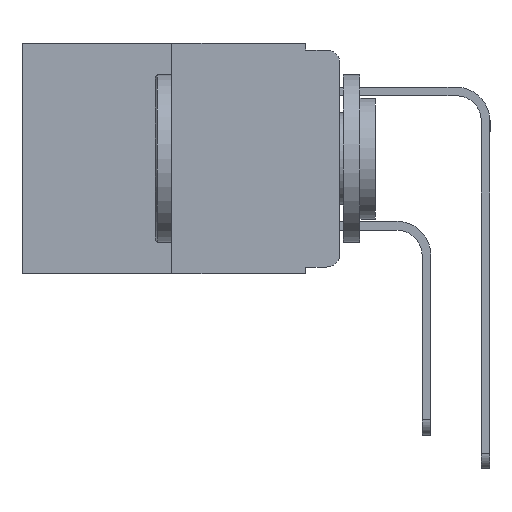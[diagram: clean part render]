
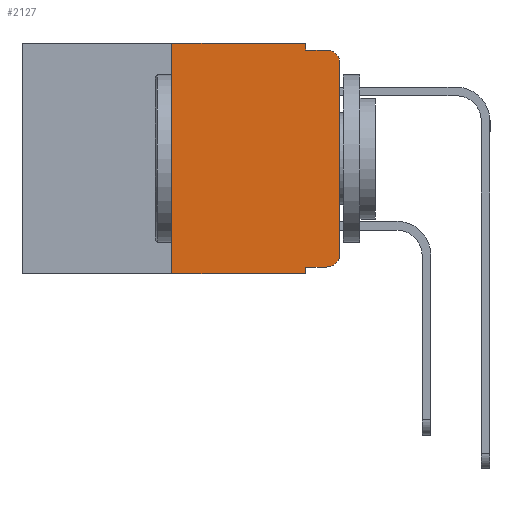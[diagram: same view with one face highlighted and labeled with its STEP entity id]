
A CAD part, left-side view. The second image highlights one B-rep face of the part: STEP entity #2127.
In plain terms, the highlighted planar face has unit normal (-1, 0, 0).
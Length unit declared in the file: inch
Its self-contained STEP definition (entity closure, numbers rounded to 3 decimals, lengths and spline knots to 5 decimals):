
#459 = VECTOR ( 'NONE', #6215, 39.37008 ) ;
#470 = VECTOR ( 'NONE', #4532, 39.37008 ) ;
#555 = EDGE_CURVE ( 'NONE', #13656, #2213, #9569, .T. ) ;
#850 = VECTOR ( 'NONE', #9833, 39.37008 ) ;
#875 = DIRECTION ( 'NONE',  ( 0., 0., -1. ) ) ;
#963 = DIRECTION ( 'NONE',  ( 0., 0., -1. ) ) ;
#992 = CARTESIAN_POINT ( 'NONE',  ( 0., 0.051, -0.01 ) ) ;
#1230 = ORIENTED_EDGE ( 'NONE', *, *, #10964, .F. ) ;
#1319 = ORIENTED_EDGE ( 'NONE', *, *, #9535, .T. ) ;
#1348 = ORIENTED_EDGE ( 'NONE', *, *, #10260, .F. ) ;
#1674 = LINE ( 'NONE', #11668, #7772 ) ;
#1982 = AXIS2_PLACEMENT_3D ( 'NONE', #13988, #7801, #875 ) ;
#2127 = ADVANCED_FACE ( 'NONE', ( #6171 ), #11903, .F. ) ;
#2213 = VERTEX_POINT ( 'NONE', #8237 ) ;
#2452 = LINE ( 'NONE', #5250, #13628 ) ;
#2521 = CARTESIAN_POINT ( 'NONE',  ( 0., 0.051, -0.333 ) ) ;
#2648 = ORIENTED_EDGE ( 'NONE', *, *, #555, .T. ) ;
#2690 = ORIENTED_EDGE ( 'NONE', *, *, #8818, .T. ) ;
#2891 = VERTEX_POINT ( 'NONE', #10440 ) ;
#2963 = VERTEX_POINT ( 'NONE', #10147 ) ;
#3169 = CARTESIAN_POINT ( 'NONE',  ( 0., 0.473, 0. ) ) ;
#3643 = VERTEX_POINT ( 'NONE', #12414 ) ;
#3748 = AXIS2_PLACEMENT_3D ( 'NONE', #14054, #7883, #963 ) ;
#4174 = CARTESIAN_POINT ( 'NONE',  ( 0., 0., -0.313 ) ) ;
#4399 = LINE ( 'NONE', #3169, #850 ) ;
#4422 = LINE ( 'NONE', #6981, #7045 ) ;
#4532 = DIRECTION ( 'NONE',  ( 0., -1., 0. ) ) ;
#4603 = CARTESIAN_POINT ( 'NONE',  ( 0., 0.25, 0. ) ) ;
#4825 = CARTESIAN_POINT ( 'NONE',  ( 0., 0.02, -0.333 ) ) ;
#4861 = ORIENTED_EDGE ( 'NONE', *, *, #12292, .F. ) ;
#5182 = DIRECTION ( 'NONE',  ( 0., 0., -1. ) ) ;
#5250 = CARTESIAN_POINT ( 'NONE',  ( 0., 0.051, -0.333 ) ) ;
#5542 = ORIENTED_EDGE ( 'NONE', *, *, #12956, .T. ) ;
#5686 = EDGE_LOOP ( 'NONE', ( #6267, #5542, #4861, #9204, #11367, #1230, #2648, #1348, #1319, #2690 ) ) ;
#5704 = CARTESIAN_POINT ( 'NONE',  ( 0., 0.473, -0.343 ) ) ;
#5944 = AXIS2_PLACEMENT_3D ( 'NONE', #9062, #13264, #13259 ) ;
#6120 = DIRECTION ( 'NONE',  ( 0., 0., 1. ) ) ;
#6171 = FACE_OUTER_BOUND ( 'NONE', #5686, .T. ) ;
#6215 = DIRECTION ( 'NONE',  ( 0., -1., 0. ) ) ;
#6267 = ORIENTED_EDGE ( 'NONE', *, *, #13649, .T. ) ;
#6360 = VERTEX_POINT ( 'NONE', #4174 ) ;
#6499 = DIRECTION ( 'NONE',  ( 0., 0., 1. ) ) ;
#6612 = VERTEX_POINT ( 'NONE', #4603 ) ;
#6735 = VERTEX_POINT ( 'NONE', #2521 ) ;
#6981 = CARTESIAN_POINT ( 'NONE',  ( 0., 0.051, 0. ) ) ;
#7045 = VECTOR ( 'NONE', #11262, 39.37008 ) ;
#7772 = VECTOR ( 'NONE', #5182, 39.37008 ) ;
#7801 = DIRECTION ( 'NONE',  ( -1., 0., 0. ) ) ;
#7883 = DIRECTION ( 'NONE',  ( -1., 0., 0. ) ) ;
#8237 = CARTESIAN_POINT ( 'NONE',  ( 0., 0.051, -0.343 ) ) ;
#8638 = CARTESIAN_POINT ( 'NONE',  ( 0., 0., -0.03 ) ) ;
#8808 = CIRCLE ( 'NONE', #3748, 0.02 ) ;
#8818 = EDGE_CURVE ( 'NONE', #10871, #6360, #8808, .T. ) ;
#8891 = CIRCLE ( 'NONE', #1982, 0.02 ) ;
#9062 = CARTESIAN_POINT ( 'NONE',  ( 0., 0.473, 0. ) ) ;
#9204 = ORIENTED_EDGE ( 'NONE', *, *, #11642, .F. ) ;
#9535 = EDGE_CURVE ( 'NONE', #6735, #10871, #2452, .T. ) ;
#9569 = LINE ( 'NONE', #5704, #459 ) ;
#9833 = DIRECTION ( 'NONE',  ( 0., -1., 0. ) ) ;
#10147 = CARTESIAN_POINT ( 'NONE',  ( 0., 0.02, -0.01 ) ) ;
#10260 = EDGE_CURVE ( 'NONE', #6735, #2213, #1674, .T. ) ;
#10440 = CARTESIAN_POINT ( 'NONE',  ( 0., 0.051, -0.01 ) ) ;
#10460 = CARTESIAN_POINT ( 'NONE',  ( 0., 0.25, 0. ) ) ;
#10871 = VERTEX_POINT ( 'NONE', #4825 ) ;
#10964 = EDGE_CURVE ( 'NONE', #13656, #6612, #13276, .T. ) ;
#11193 = VERTEX_POINT ( 'NONE', #8638 ) ;
#11224 = VECTOR ( 'NONE', #6499, 39.37008 ) ;
#11262 = DIRECTION ( 'NONE',  ( 0., 0., -1. ) ) ;
#11367 = ORIENTED_EDGE ( 'NONE', *, *, #12884, .F. ) ;
#11543 = LINE ( 'NONE', #11844, #11224 ) ;
#11642 = EDGE_CURVE ( 'NONE', #3643, #2891, #4422, .T. ) ;
#11668 = CARTESIAN_POINT ( 'NONE',  ( 0., 0.051, 0. ) ) ;
#11723 = DIRECTION ( 'NONE',  ( 0., -1., 0. ) ) ;
#11844 = CARTESIAN_POINT ( 'NONE',  ( 0., 0., 0. ) ) ;
#11903 = PLANE ( 'NONE',  #5944 ) ;
#12292 = EDGE_CURVE ( 'NONE', #2891, #2963, #12310, .T. ) ;
#12310 = LINE ( 'NONE', #992, #470 ) ;
#12414 = CARTESIAN_POINT ( 'NONE',  ( 0., 0.051, 0. ) ) ;
#12836 = CARTESIAN_POINT ( 'NONE',  ( 0., 0.25, -0.343 ) ) ;
#12884 = EDGE_CURVE ( 'NONE', #6612, #3643, #4399, .T. ) ;
#12956 = EDGE_CURVE ( 'NONE', #11193, #2963, #8891, .T. ) ;
#12959 = VECTOR ( 'NONE', #6120, 39.37008 ) ;
#13259 = DIRECTION ( 'NONE',  ( 0., 0., -1. ) ) ;
#13264 = DIRECTION ( 'NONE',  ( 1., 0., 0. ) ) ;
#13276 = LINE ( 'NONE', #10460, #12959 ) ;
#13628 = VECTOR ( 'NONE', #11723, 39.37008 ) ;
#13649 = EDGE_CURVE ( 'NONE', #6360, #11193, #11543, .T. ) ;
#13656 = VERTEX_POINT ( 'NONE', #12836 ) ;
#13988 = CARTESIAN_POINT ( 'NONE',  ( 0., 0.02, -0.03 ) ) ;
#14054 = CARTESIAN_POINT ( 'NONE',  ( 0., 0.02, -0.313 ) ) ;
